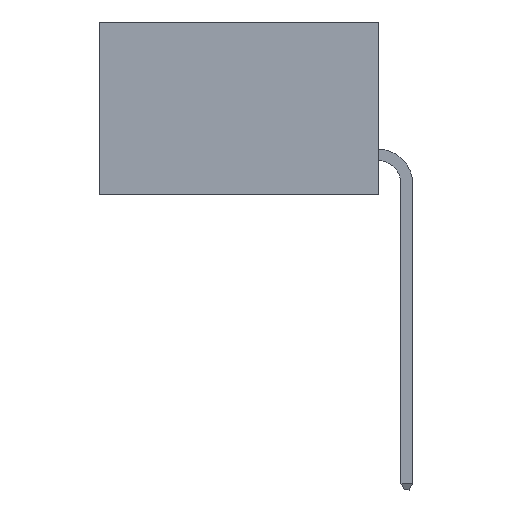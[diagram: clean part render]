
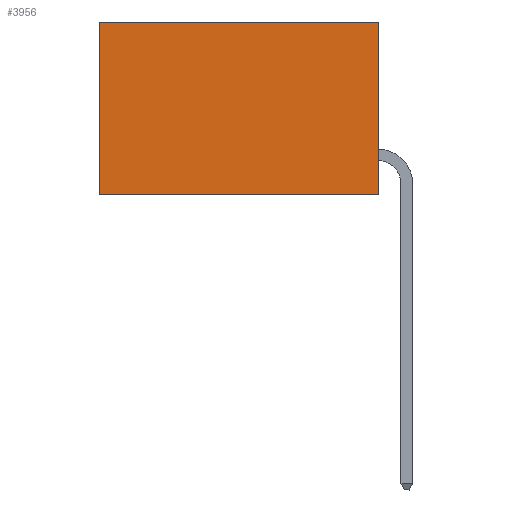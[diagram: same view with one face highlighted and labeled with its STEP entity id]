
A CAD part, left-side view. The second image highlights one B-rep face of the part: STEP entity #3956.
In plain terms, the highlighted planar face has unit normal (-1, 0, 0).
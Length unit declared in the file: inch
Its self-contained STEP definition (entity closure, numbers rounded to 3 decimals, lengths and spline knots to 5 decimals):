
#476 = LINE ( 'NONE', #15620, #15215 ) ;
#2113 = CARTESIAN_POINT ( 'NONE',  ( 0.2615, 0., -0.37 ) ) ;
#3846 = VECTOR ( 'NONE', #17279, 39.37008 ) ;
#3956 = ADVANCED_FACE ( 'NONE', ( #14119 ), #23020, .F. ) ;
#3986 = DIRECTION ( 'NONE',  ( 0., 0., -1. ) ) ;
#4092 = CARTESIAN_POINT ( 'NONE',  ( 0.2615, 0., -0.37 ) ) ;
#4167 = EDGE_LOOP ( 'NONE', ( #21564, #18454, #4416, #22078 ) ) ;
#4416 = ORIENTED_EDGE ( 'NONE', *, *, #7833, .F. ) ;
#4651 = DIRECTION ( 'NONE',  ( 0., 0., -1. ) ) ;
#5120 = DIRECTION ( 'NONE',  ( 0., 0., -1. ) ) ;
#6078 = VERTEX_POINT ( 'NONE', #13714 ) ;
#7833 = EDGE_CURVE ( 'NONE', #9073, #10109, #13555, .T. ) ;
#7922 = VERTEX_POINT ( 'NONE', #17898 ) ;
#8002 = CARTESIAN_POINT ( 'NONE',  ( 0.2615, 0., -0.37 ) ) ;
#8049 = DIRECTION ( 'NONE',  ( 0., 1., 0. ) ) ;
#9073 = VERTEX_POINT ( 'NONE', #9695 ) ;
#9508 = AXIS2_PLACEMENT_3D ( 'NONE', #8002, #21663, #4651 ) ;
#9695 = CARTESIAN_POINT ( 'NONE',  ( 0.2615, 0., 0. ) ) ;
#10109 = VERTEX_POINT ( 'NONE', #16835 ) ;
#11542 = LINE ( 'NONE', #2113, #3846 ) ;
#12092 = VECTOR ( 'NONE', #5120, 39.37008 ) ;
#13555 = LINE ( 'NONE', #4092, #20394 ) ;
#13714 = CARTESIAN_POINT ( 'NONE',  ( 0.2615, 0.6, -0.37 ) ) ;
#14119 = FACE_OUTER_BOUND ( 'NONE', #4167, .T. ) ;
#15044 = CARTESIAN_POINT ( 'NONE',  ( 0.2615, 0.6, -0.37 ) ) ;
#15215 = VECTOR ( 'NONE', #8049, 39.37008 ) ;
#15620 = CARTESIAN_POINT ( 'NONE',  ( 0.2615, 0., 0. ) ) ;
#16835 = CARTESIAN_POINT ( 'NONE',  ( 0.2615, 0., -0.37 ) ) ;
#17279 = DIRECTION ( 'NONE',  ( 0., 1., 0. ) ) ;
#17898 = CARTESIAN_POINT ( 'NONE',  ( 0.2615, 0.6, 0. ) ) ;
#18454 = ORIENTED_EDGE ( 'NONE', *, *, #22831, .F. ) ;
#19300 = EDGE_CURVE ( 'NONE', #9073, #7922, #476, .T. ) ;
#20277 = EDGE_CURVE ( 'NONE', #7922, #6078, #20416, .T. ) ;
#20394 = VECTOR ( 'NONE', #3986, 39.37008 ) ;
#20416 = LINE ( 'NONE', #15044, #12092 ) ;
#21564 = ORIENTED_EDGE ( 'NONE', *, *, #20277, .T. ) ;
#21663 = DIRECTION ( 'NONE',  ( 1., 0., 0. ) ) ;
#22078 = ORIENTED_EDGE ( 'NONE', *, *, #19300, .T. ) ;
#22831 = EDGE_CURVE ( 'NONE', #10109, #6078, #11542, .T. ) ;
#23020 = PLANE ( 'NONE',  #9508 ) ;
